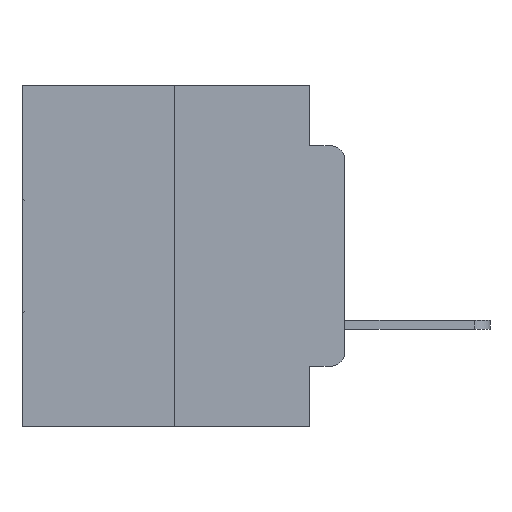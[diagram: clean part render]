
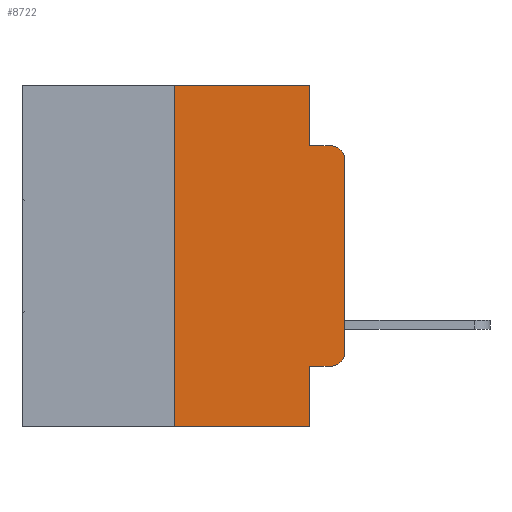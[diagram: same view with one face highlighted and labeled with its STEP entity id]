
A CAD part, left-side view. The second image highlights one B-rep face of the part: STEP entity #8722.
In plain terms, the highlighted planar face has unit normal (-1, 0, 0).
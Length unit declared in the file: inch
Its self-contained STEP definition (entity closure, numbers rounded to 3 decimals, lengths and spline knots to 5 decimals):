
#649 = DIRECTION ( 'NONE',  ( 0., -1., 0. ) ) ;
#896 = ORIENTED_EDGE ( 'NONE', *, *, #19275, .F. ) ;
#2276 = ORIENTED_EDGE ( 'NONE', *, *, #23729, .T. ) ;
#2397 = EDGE_CURVE ( 'NONE', #17479, #20579, #19791, .T. ) ;
#2858 = EDGE_CURVE ( 'NONE', #18751, #11497, #15097, .T. ) ;
#4494 = DIRECTION ( 'NONE',  ( 0., 0., 1. ) ) ;
#4546 = ORIENTED_EDGE ( 'NONE', *, *, #2397, .T. ) ;
#4565 = CARTESIAN_POINT ( 'NONE',  ( 0., 0.051, -0.4115 ) ) ;
#4572 = EDGE_CURVE ( 'NONE', #12468, #7044, #28497, .T. ) ;
#5103 = CARTESIAN_POINT ( 'NONE',  ( 0., 0.02, -0.4115 ) ) ;
#5396 = VECTOR ( 'NONE', #27383, 39.37008 ) ;
#5449 = CARTESIAN_POINT ( 'NONE',  ( 0., 0.02, -0.0885 ) ) ;
#5498 = CARTESIAN_POINT ( 'NONE',  ( 0., 0., -0.1085 ) ) ;
#5682 = LINE ( 'NONE', #14579, #6414 ) ;
#6414 = VECTOR ( 'NONE', #25903, 39.37008 ) ;
#6857 = LINE ( 'NONE', #24201, #27059 ) ;
#7044 = VERTEX_POINT ( 'NONE', #27981 ) ;
#7183 = EDGE_CURVE ( 'NONE', #11497, #17639, #5682, .T. ) ;
#7263 = VECTOR ( 'NONE', #13336, 39.37008 ) ;
#7793 = CARTESIAN_POINT ( 'NONE',  ( 0., 0.473, 0. ) ) ;
#7845 = CARTESIAN_POINT ( 'NONE',  ( 0., 0.051, -0.4115 ) ) ;
#7934 = DIRECTION ( 'NONE',  ( 0., -1., 0. ) ) ;
#8181 = CARTESIAN_POINT ( 'NONE',  ( 0., 0.25, -0.5 ) ) ;
#8332 = ORIENTED_EDGE ( 'NONE', *, *, #2858, .F. ) ;
#8458 = DIRECTION ( 'NONE',  ( 0., 0., -1. ) ) ;
#8722 = ADVANCED_FACE ( 'NONE', ( #11553 ), #17482, .F. ) ;
#9041 = CARTESIAN_POINT ( 'NONE',  ( 0., 0.25, 0. ) ) ;
#9074 = VERTEX_POINT ( 'NONE', #8181 ) ;
#9567 = VECTOR ( 'NONE', #649, 39.37008 ) ;
#9744 = VECTOR ( 'NONE', #7934, 39.37008 ) ;
#10279 = DIRECTION ( 'NONE',  ( 0., -1., 0. ) ) ;
#10518 = DIRECTION ( 'NONE',  ( 0., 0., 1. ) ) ;
#11497 = VERTEX_POINT ( 'NONE', #25969 ) ;
#11513 = CARTESIAN_POINT ( 'NONE',  ( 0., 0.051, 0. ) ) ;
#11553 = FACE_OUTER_BOUND ( 'NONE', #22828, .T. ) ;
#11635 = DIRECTION ( 'NONE',  ( -1., 0., 0. ) ) ;
#12007 = ORIENTED_EDGE ( 'NONE', *, *, #4572, .T. ) ;
#12262 = EDGE_CURVE ( 'NONE', #17639, #20579, #13801, .T. ) ;
#12468 = VERTEX_POINT ( 'NONE', #5103 ) ;
#12979 = CARTESIAN_POINT ( 'NONE',  ( 0., 0.473, 0. ) ) ;
#13288 = LINE ( 'NONE', #13429, #7263 ) ;
#13336 = DIRECTION ( 'NONE',  ( 0., -1., 0. ) ) ;
#13429 = CARTESIAN_POINT ( 'NONE',  ( 0., 0.473, -0.5 ) ) ;
#13801 = LINE ( 'NONE', #18110, #9567 ) ;
#14256 = ORIENTED_EDGE ( 'NONE', *, *, #7183, .F. ) ;
#14579 = CARTESIAN_POINT ( 'NONE',  ( 0., 0.051, 0. ) ) ;
#15097 = LINE ( 'NONE', #7793, #15479 ) ;
#15479 = VECTOR ( 'NONE', #10279, 39.37008 ) ;
#15572 = EDGE_CURVE ( 'NONE', #19510, #12468, #15780, .T. ) ;
#15780 = LINE ( 'NONE', #7845, #9744 ) ;
#16008 = VERTEX_POINT ( 'NONE', #28545 ) ;
#17206 = EDGE_CURVE ( 'NONE', #7044, #17479, #6857, .T. ) ;
#17309 = AXIS2_PLACEMENT_3D ( 'NONE', #12979, #17800, #8458 ) ;
#17479 = VERTEX_POINT ( 'NONE', #5498 ) ;
#17482 = PLANE ( 'NONE',  #17309 ) ;
#17622 = CARTESIAN_POINT ( 'NONE',  ( 0., 0.25, 0. ) ) ;
#17639 = VERTEX_POINT ( 'NONE', #27272 ) ;
#17800 = DIRECTION ( 'NONE',  ( 1., 0., 0. ) ) ;
#18110 = CARTESIAN_POINT ( 'NONE',  ( 0., 0.051, -0.0885 ) ) ;
#18581 = ORIENTED_EDGE ( 'NONE', *, *, #17206, .T. ) ;
#18751 = VERTEX_POINT ( 'NONE', #17622 ) ;
#19078 = ORIENTED_EDGE ( 'NONE', *, *, #12262, .F. ) ;
#19275 = EDGE_CURVE ( 'NONE', #19510, #16008, #21022, .T. ) ;
#19508 = LINE ( 'NONE', #9041, #26568 ) ;
#19510 = VERTEX_POINT ( 'NONE', #4565 ) ;
#19791 = CIRCLE ( 'NONE', #19925, 0.02 ) ;
#19925 = AXIS2_PLACEMENT_3D ( 'NONE', #25251, #11635, #20883 ) ;
#20214 = DIRECTION ( 'NONE',  ( 0., 0., -1. ) ) ;
#20579 = VERTEX_POINT ( 'NONE', #5449 ) ;
#20883 = DIRECTION ( 'NONE',  ( 0., 0., -1. ) ) ;
#21022 = LINE ( 'NONE', #11513, #5396 ) ;
#22615 = CARTESIAN_POINT ( 'NONE',  ( 0., 0.02, -0.3915 ) ) ;
#22828 = EDGE_LOOP ( 'NONE', ( #18581, #4546, #19078, #14256, #8332, #24080, #2276, #896, #27434, #12007 ) ) ;
#23729 = EDGE_CURVE ( 'NONE', #9074, #16008, #13288, .T. ) ;
#23781 = AXIS2_PLACEMENT_3D ( 'NONE', #22615, #29300, #20214 ) ;
#24080 = ORIENTED_EDGE ( 'NONE', *, *, #29050, .F. ) ;
#24201 = CARTESIAN_POINT ( 'NONE',  ( 0., 0., 0. ) ) ;
#25251 = CARTESIAN_POINT ( 'NONE',  ( 0., 0.02, -0.1085 ) ) ;
#25903 = DIRECTION ( 'NONE',  ( 0., 0., -1. ) ) ;
#25969 = CARTESIAN_POINT ( 'NONE',  ( 0., 0.051, 0. ) ) ;
#26568 = VECTOR ( 'NONE', #4494, 39.37008 ) ;
#27059 = VECTOR ( 'NONE', #10518, 39.37008 ) ;
#27272 = CARTESIAN_POINT ( 'NONE',  ( 0., 0.051, -0.0885 ) ) ;
#27383 = DIRECTION ( 'NONE',  ( 0., 0., -1. ) ) ;
#27434 = ORIENTED_EDGE ( 'NONE', *, *, #15572, .T. ) ;
#27981 = CARTESIAN_POINT ( 'NONE',  ( 0., 0., -0.3915 ) ) ;
#28497 = CIRCLE ( 'NONE', #23781, 0.02 ) ;
#28545 = CARTESIAN_POINT ( 'NONE',  ( 0., 0.051, -0.5 ) ) ;
#29050 = EDGE_CURVE ( 'NONE', #9074, #18751, #19508, .T. ) ;
#29300 = DIRECTION ( 'NONE',  ( -1., 0., 0. ) ) ;
